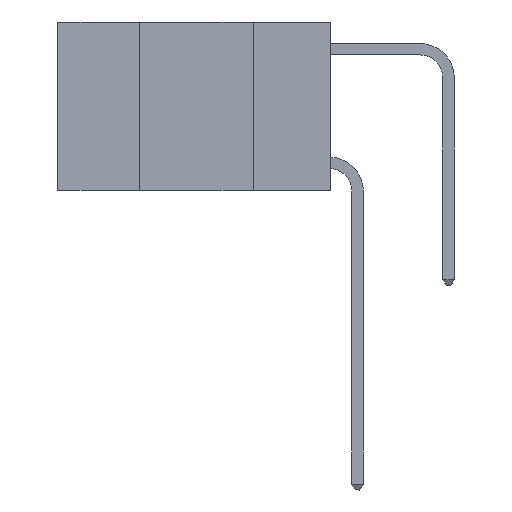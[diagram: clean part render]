
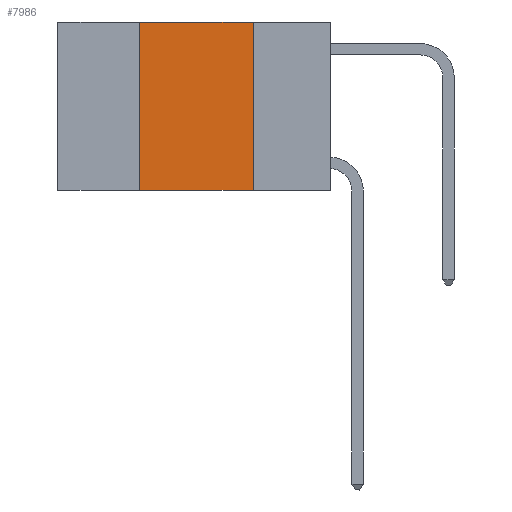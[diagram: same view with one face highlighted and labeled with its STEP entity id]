
A CAD part, left-side view. The second image highlights one B-rep face of the part: STEP entity #7986.
In plain terms, the highlighted planar face has unit normal (-1, 0, 0).
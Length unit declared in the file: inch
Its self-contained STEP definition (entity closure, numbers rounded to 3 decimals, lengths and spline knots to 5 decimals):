
#238 = LINE ( 'NONE', #21018, #14731 ) ;
#265 = CARTESIAN_POINT ( 'NONE',  ( 0., 0.17, 0. ) ) ;
#1084 = PLANE ( 'NONE',  #3374 ) ;
#1304 = VERTEX_POINT ( 'NONE', #11713 ) ;
#2187 = CARTESIAN_POINT ( 'NONE',  ( 0., 0.42, -0.37 ) ) ;
#3374 = AXIS2_PLACEMENT_3D ( 'NONE', #20867, #31123, #16037 ) ;
#3635 = VERTEX_POINT ( 'NONE', #2187 ) ;
#4449 = EDGE_CURVE ( 'NONE', #3635, #1304, #13416, .T. ) ;
#4565 = CARTESIAN_POINT ( 'NONE',  ( 0., 0.6, -0.37 ) ) ;
#4966 = ORIENTED_EDGE ( 'NONE', *, *, #26450, .F. ) ;
#6453 = VECTOR ( 'NONE', #29721, 39.37008 ) ;
#7131 = ORIENTED_EDGE ( 'NONE', *, *, #28232, .F. ) ;
#7287 = FACE_OUTER_BOUND ( 'NONE', #16431, .T. ) ;
#7986 = ADVANCED_FACE ( 'NONE', ( #7287 ), #1084, .F. ) ;
#8630 = VECTOR ( 'NONE', #30267, 39.37008 ) ;
#11051 = EDGE_CURVE ( 'NONE', #19284, #1304, #26994, .T. ) ;
#11713 = CARTESIAN_POINT ( 'NONE',  ( 0., 0.17, -0.37 ) ) ;
#13416 = LINE ( 'NONE', #4565, #6453 ) ;
#14731 = VECTOR ( 'NONE', #23290, 39.37008 ) ;
#15058 = CARTESIAN_POINT ( 'NONE',  ( 0., 0.6, 0. ) ) ;
#16037 = DIRECTION ( 'NONE',  ( 0., 0., -1. ) ) ;
#16431 = EDGE_LOOP ( 'NONE', ( #22717, #4966, #7131, #18108 ) ) ;
#16753 = VECTOR ( 'NONE', #24654, 39.37008 ) ;
#18108 = ORIENTED_EDGE ( 'NONE', *, *, #4449, .T. ) ;
#19284 = VERTEX_POINT ( 'NONE', #265 ) ;
#19896 = CARTESIAN_POINT ( 'NONE',  ( 0., 0.17, 0. ) ) ;
#20705 = LINE ( 'NONE', #15058, #8630 ) ;
#20867 = CARTESIAN_POINT ( 'NONE',  ( 0., 0.6, 0. ) ) ;
#21018 = CARTESIAN_POINT ( 'NONE',  ( 0., 0.42, 0. ) ) ;
#22717 = ORIENTED_EDGE ( 'NONE', *, *, #11051, .F. ) ;
#23290 = DIRECTION ( 'NONE',  ( 0., 0., 1. ) ) ;
#24271 = CARTESIAN_POINT ( 'NONE',  ( 0., 0.42, 0. ) ) ;
#24654 = DIRECTION ( 'NONE',  ( 0., 0., -1. ) ) ;
#26450 = EDGE_CURVE ( 'NONE', #29252, #19284, #20705, .T. ) ;
#26994 = LINE ( 'NONE', #19896, #16753 ) ;
#28232 = EDGE_CURVE ( 'NONE', #3635, #29252, #238, .T. ) ;
#29252 = VERTEX_POINT ( 'NONE', #24271 ) ;
#29721 = DIRECTION ( 'NONE',  ( 0., -1., 0. ) ) ;
#30267 = DIRECTION ( 'NONE',  ( 0., -1., 0. ) ) ;
#31123 = DIRECTION ( 'NONE',  ( 1., 0., 0. ) ) ;
